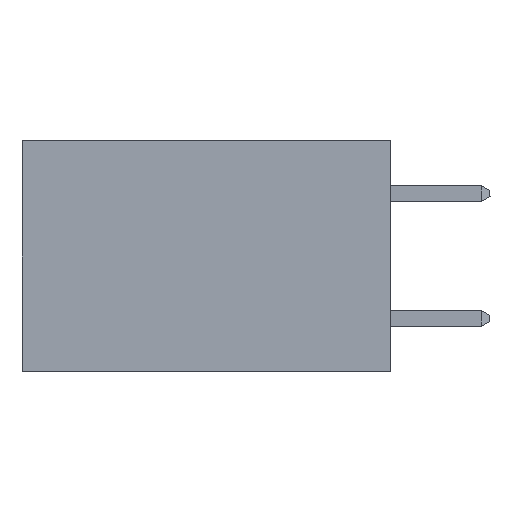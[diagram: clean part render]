
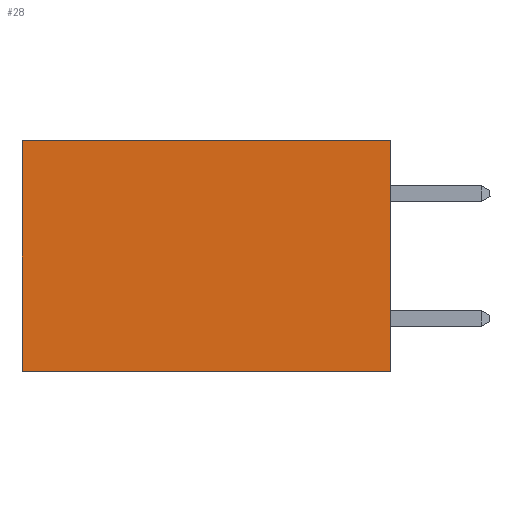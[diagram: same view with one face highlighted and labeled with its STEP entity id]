
A CAD part, left-side view. The second image highlights one B-rep face of the part: STEP entity #28.
In plain terms, the highlighted planar face has unit normal (-1, 0, 0).
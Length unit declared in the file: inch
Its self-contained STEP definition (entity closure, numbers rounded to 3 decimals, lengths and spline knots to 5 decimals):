
#28 = ADVANCED_FACE ( 'NONE', ( #10141 ), #732, .F. ) ;
#124 = VERTEX_POINT ( 'NONE', #21070 ) ;
#649 = VERTEX_POINT ( 'NONE', #16418 ) ;
#732 = PLANE ( 'NONE',  #10908 ) ;
#879 = DIRECTION ( 'NONE',  ( 0., 0., -1. ) ) ;
#1604 = DIRECTION ( 'NONE',  ( 0., 0., -1. ) ) ;
#2028 = EDGE_LOOP ( 'NONE', ( #22662, #21937, #7838, #24227 ) ) ;
#2424 = CARTESIAN_POINT ( 'NONE',  ( 0.277, 0.59, -0.37 ) ) ;
#5729 = CARTESIAN_POINT ( 'NONE',  ( 0.277, 0., -0.37 ) ) ;
#7838 = ORIENTED_EDGE ( 'NONE', *, *, #25190, .F. ) ;
#8101 = EDGE_CURVE ( 'NONE', #25035, #23582, #29960, .T. ) ;
#8472 = CARTESIAN_POINT ( 'NONE',  ( 0.277, 0., 0. ) ) ;
#9174 = CARTESIAN_POINT ( 'NONE',  ( 0.277, 0., -0.37 ) ) ;
#9203 = DIRECTION ( 'NONE',  ( 0., 1., 0. ) ) ;
#9713 = VECTOR ( 'NONE', #17629, 39.37008 ) ;
#10141 = FACE_OUTER_BOUND ( 'NONE', #2028, .T. ) ;
#10908 = AXIS2_PLACEMENT_3D ( 'NONE', #9174, #12865, #1604 ) ;
#11074 = DIRECTION ( 'NONE',  ( 0., 0., -1. ) ) ;
#11538 = CARTESIAN_POINT ( 'NONE',  ( 0.277, 0.59, -0.37 ) ) ;
#12865 = DIRECTION ( 'NONE',  ( 1., 0., 0. ) ) ;
#13169 = VECTOR ( 'NONE', #879, 39.37008 ) ;
#15985 = VECTOR ( 'NONE', #9203, 39.37008 ) ;
#16166 = LINE ( 'NONE', #8472, #9713 ) ;
#16275 = EDGE_CURVE ( 'NONE', #649, #23582, #17468, .T. ) ;
#16418 = CARTESIAN_POINT ( 'NONE',  ( 0.277, 0., -0.37 ) ) ;
#16420 = CARTESIAN_POINT ( 'NONE',  ( 0.277, 0., -0.37 ) ) ;
#17468 = LINE ( 'NONE', #16420, #15985 ) ;
#17629 = DIRECTION ( 'NONE',  ( 0., 1., 0. ) ) ;
#19756 = CARTESIAN_POINT ( 'NONE',  ( 0.277, 0.59, 0. ) ) ;
#20338 = LINE ( 'NONE', #5729, #13169 ) ;
#21070 = CARTESIAN_POINT ( 'NONE',  ( 0.277, 0., 0. ) ) ;
#21937 = ORIENTED_EDGE ( 'NONE', *, *, #16275, .F. ) ;
#22464 = EDGE_CURVE ( 'NONE', #124, #25035, #16166, .T. ) ;
#22662 = ORIENTED_EDGE ( 'NONE', *, *, #8101, .T. ) ;
#23582 = VERTEX_POINT ( 'NONE', #2424 ) ;
#24227 = ORIENTED_EDGE ( 'NONE', *, *, #22464, .T. ) ;
#25035 = VERTEX_POINT ( 'NONE', #19756 ) ;
#25190 = EDGE_CURVE ( 'NONE', #124, #649, #20338, .T. ) ;
#29227 = VECTOR ( 'NONE', #11074, 39.37008 ) ;
#29960 = LINE ( 'NONE', #11538, #29227 ) ;
